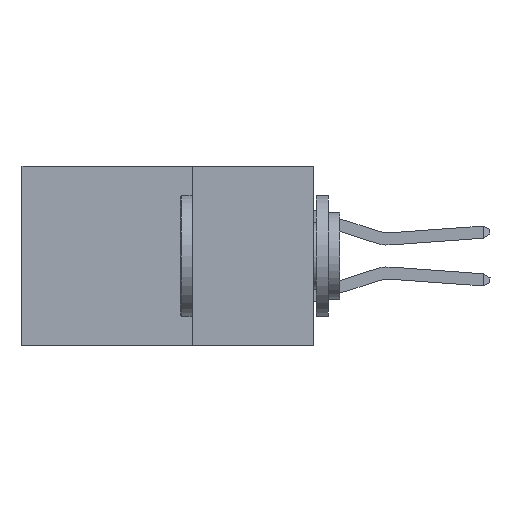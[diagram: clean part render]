
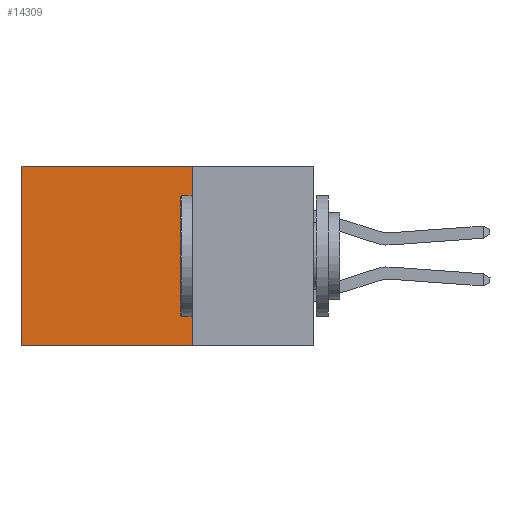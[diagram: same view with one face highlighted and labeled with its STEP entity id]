
A CAD part, left-side view. The second image highlights one B-rep face of the part: STEP entity #14309.
In plain terms, the highlighted planar face has unit normal (-1, 0, 0).
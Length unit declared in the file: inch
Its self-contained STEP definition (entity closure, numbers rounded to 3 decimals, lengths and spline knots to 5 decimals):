
#16 = VERTEX_POINT ( 'NONE', #14410 ) ;
#1623 = ORIENTED_EDGE ( 'NONE', *, *, #3625, .T. ) ;
#2613 = VECTOR ( 'NONE', #16424, 39.37008 ) ;
#3535 = ORIENTED_EDGE ( 'NONE', *, *, #12879, .F. ) ;
#3625 = EDGE_CURVE ( 'NONE', #16, #8905, #7226, .T. ) ;
#3814 = DIRECTION ( 'NONE',  ( 0., 0., -1. ) ) ;
#3891 = CARTESIAN_POINT ( 'NONE',  ( 0.2875, 0.6, 0. ) ) ;
#4767 = CARTESIAN_POINT ( 'NONE',  ( 0.2875, 0.25, -0.37 ) ) ;
#5624 = DIRECTION ( 'NONE',  ( 0., 0., -1. ) ) ;
#5682 = PLANE ( 'NONE',  #7573 ) ;
#6094 = VECTOR ( 'NONE', #16573, 39.37008 ) ;
#7226 = LINE ( 'NONE', #3891, #19599 ) ;
#7366 = CARTESIAN_POINT ( 'NONE',  ( 0.2875, 0.25, 0. ) ) ;
#7451 = VERTEX_POINT ( 'NONE', #19486 ) ;
#7573 = AXIS2_PLACEMENT_3D ( 'NONE', #7366, #19112, #9076 ) ;
#8905 = VERTEX_POINT ( 'NONE', #13539 ) ;
#9076 = DIRECTION ( 'NONE',  ( 0., 0., -1. ) ) ;
#9249 = FACE_OUTER_BOUND ( 'NONE', #16519, .T. ) ;
#10561 = LINE ( 'NONE', #4767, #6094 ) ;
#11606 = LINE ( 'NONE', #14731, #2613 ) ;
#11811 = VERTEX_POINT ( 'NONE', #20733 ) ;
#12879 = EDGE_CURVE ( 'NONE', #11811, #7451, #15095, .T. ) ;
#13112 = ORIENTED_EDGE ( 'NONE', *, *, #14072, .F. ) ;
#13539 = CARTESIAN_POINT ( 'NONE',  ( 0.2875, 0.6, -0.37 ) ) ;
#13928 = CARTESIAN_POINT ( 'NONE',  ( 0.2875, 0.25, 0. ) ) ;
#14013 = EDGE_CURVE ( 'NONE', #11811, #16, #11606, .T. ) ;
#14072 = EDGE_CURVE ( 'NONE', #7451, #8905, #10561, .T. ) ;
#14309 = ADVANCED_FACE ( 'NONE', ( #9249 ), #5682, .F. ) ;
#14410 = CARTESIAN_POINT ( 'NONE',  ( 0.2875, 0.6, 0. ) ) ;
#14731 = CARTESIAN_POINT ( 'NONE',  ( 0.2875, 0.25, 0. ) ) ;
#15095 = LINE ( 'NONE', #13928, #19565 ) ;
#16424 = DIRECTION ( 'NONE',  ( 0., 1., 0. ) ) ;
#16519 = EDGE_LOOP ( 'NONE', ( #1623, #13112, #3535, #16522 ) ) ;
#16522 = ORIENTED_EDGE ( 'NONE', *, *, #14013, .T. ) ;
#16573 = DIRECTION ( 'NONE',  ( 0., 1., 0. ) ) ;
#19112 = DIRECTION ( 'NONE',  ( 1., 0., 0. ) ) ;
#19486 = CARTESIAN_POINT ( 'NONE',  ( 0.2875, 0.25, -0.37 ) ) ;
#19565 = VECTOR ( 'NONE', #3814, 39.37008 ) ;
#19599 = VECTOR ( 'NONE', #5624, 39.37008 ) ;
#20733 = CARTESIAN_POINT ( 'NONE',  ( 0.2875, 0.25, 0. ) ) ;
